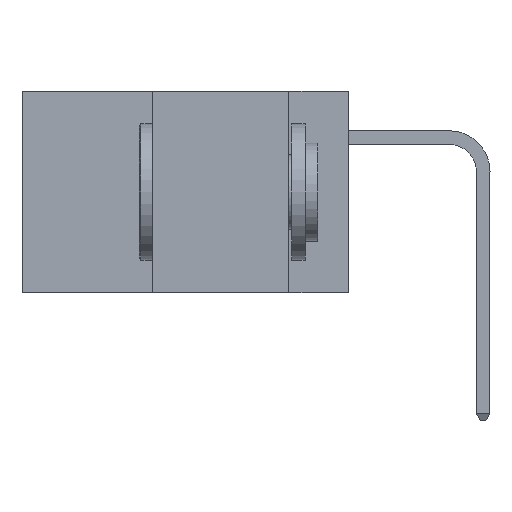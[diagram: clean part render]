
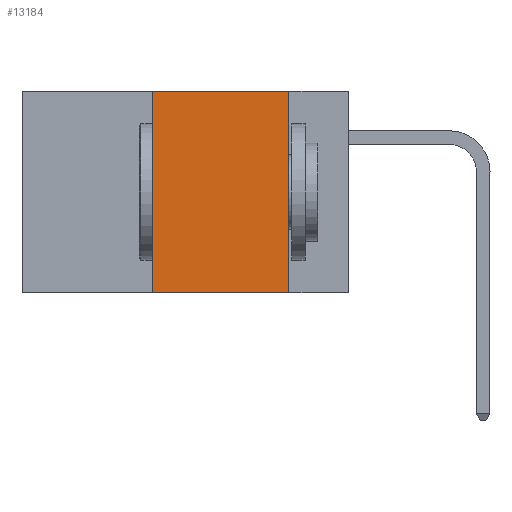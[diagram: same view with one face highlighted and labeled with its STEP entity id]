
A CAD part, left-side view. The second image highlights one B-rep face of the part: STEP entity #13184.
In plain terms, the highlighted planar face has unit normal (-1, 0, 0).
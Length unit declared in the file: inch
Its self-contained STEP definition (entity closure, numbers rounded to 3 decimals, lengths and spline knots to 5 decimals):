
#282 = ORIENTED_EDGE ( 'NONE', *, *, #8785, .F. ) ;
#847 = PLANE ( 'NONE',  #10590 ) ;
#978 = ORIENTED_EDGE ( 'NONE', *, *, #12995, .T. ) ;
#1294 = ORIENTED_EDGE ( 'NONE', *, *, #10820, .F. ) ;
#2005 = DIRECTION ( 'NONE',  ( 1., 0., 0. ) ) ;
#2571 = VECTOR ( 'NONE', #13147, 39.37008 ) ;
#3195 = LINE ( 'NONE', #14496, #5792 ) ;
#4485 = DIRECTION ( 'NONE',  ( 0., -1., 0. ) ) ;
#5326 = CARTESIAN_POINT ( 'NONE',  ( 0., 0.11, 0. ) ) ;
#5526 = CARTESIAN_POINT ( 'NONE',  ( 0., 0.36, 0. ) ) ;
#5792 = VECTOR ( 'NONE', #4485, 39.37008 ) ;
#6148 = DIRECTION ( 'NONE',  ( 0., -1., 0. ) ) ;
#6233 = CARTESIAN_POINT ( 'NONE',  ( 0., 0.36, -0.37 ) ) ;
#6251 = VECTOR ( 'NONE', #12951, 39.37008 ) ;
#7402 = CARTESIAN_POINT ( 'NONE',  ( 0., 0.11, -0.37 ) ) ;
#7613 = CARTESIAN_POINT ( 'NONE',  ( 0., 0.6, 0. ) ) ;
#7755 = VECTOR ( 'NONE', #6148, 39.37008 ) ;
#7822 = LINE ( 'NONE', #5326, #2571 ) ;
#8534 = ORIENTED_EDGE ( 'NONE', *, *, #10754, .F. ) ;
#8557 = CARTESIAN_POINT ( 'NONE',  ( 0., 0.36, 0. ) ) ;
#8785 = EDGE_CURVE ( 'NONE', #10425, #10006, #3195, .T. ) ;
#9757 = EDGE_LOOP ( 'NONE', ( #1294, #282, #8534, #978 ) ) ;
#9835 = DIRECTION ( 'NONE',  ( 0., 0., -1. ) ) ;
#10006 = VERTEX_POINT ( 'NONE', #11510 ) ;
#10342 = LINE ( 'NONE', #11703, #7755 ) ;
#10425 = VERTEX_POINT ( 'NONE', #5526 ) ;
#10590 = AXIS2_PLACEMENT_3D ( 'NONE', #7613, #2005, #9835 ) ;
#10734 = VERTEX_POINT ( 'NONE', #7402 ) ;
#10754 = EDGE_CURVE ( 'NONE', #13570, #10425, #11821, .T. ) ;
#10820 = EDGE_CURVE ( 'NONE', #10006, #10734, #7822, .T. ) ;
#11510 = CARTESIAN_POINT ( 'NONE',  ( 0., 0.11, 0. ) ) ;
#11703 = CARTESIAN_POINT ( 'NONE',  ( 0., 0.6, -0.37 ) ) ;
#11821 = LINE ( 'NONE', #8557, #6251 ) ;
#12804 = FACE_OUTER_BOUND ( 'NONE', #9757, .T. ) ;
#12951 = DIRECTION ( 'NONE',  ( 0., 0., 1. ) ) ;
#12995 = EDGE_CURVE ( 'NONE', #13570, #10734, #10342, .T. ) ;
#13147 = DIRECTION ( 'NONE',  ( 0., 0., -1. ) ) ;
#13184 = ADVANCED_FACE ( 'NONE', ( #12804 ), #847, .F. ) ;
#13570 = VERTEX_POINT ( 'NONE', #6233 ) ;
#14496 = CARTESIAN_POINT ( 'NONE',  ( 0., 0.6, 0. ) ) ;
